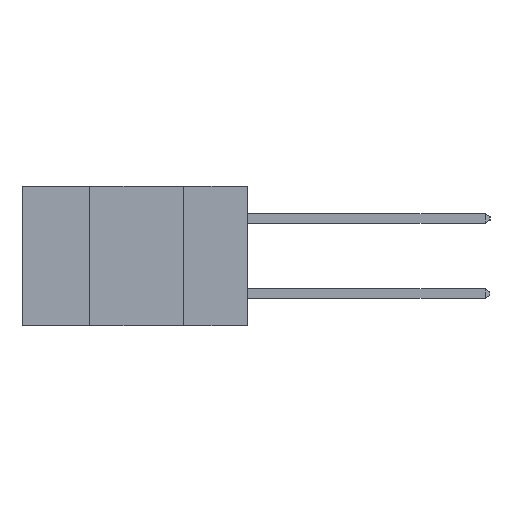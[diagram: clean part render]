
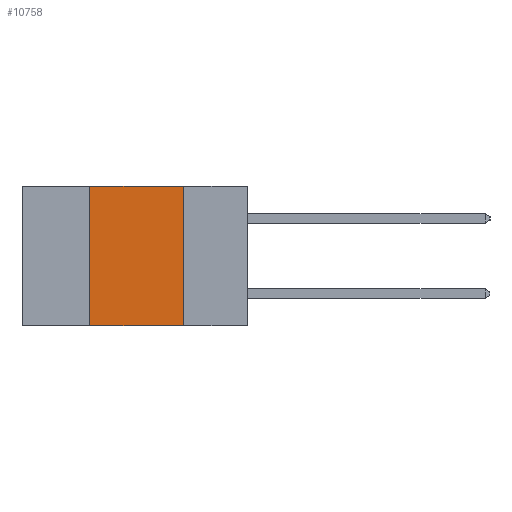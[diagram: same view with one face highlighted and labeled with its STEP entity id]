
A CAD part, left-side view. The second image highlights one B-rep face of the part: STEP entity #10758.
In plain terms, the highlighted planar face has unit normal (-1, 0, 0).
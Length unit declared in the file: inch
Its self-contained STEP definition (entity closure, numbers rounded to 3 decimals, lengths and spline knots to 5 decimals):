
#1154 = VERTEX_POINT ( 'NONE', #9420 ) ;
#1425 = CARTESIAN_POINT ( 'NONE',  ( 0., 0.17, 0. ) ) ;
#1762 = VERTEX_POINT ( 'NONE', #4291 ) ;
#2088 = CARTESIAN_POINT ( 'NONE',  ( 0., 0.42, 0. ) ) ;
#2187 = DIRECTION ( 'NONE',  ( 0., 0., 1. ) ) ;
#2316 = LINE ( 'NONE', #3023, #7748 ) ;
#2610 = LINE ( 'NONE', #6621, #13766 ) ;
#3023 = CARTESIAN_POINT ( 'NONE',  ( 0., 0.6, -0.37 ) ) ;
#3049 = ORIENTED_EDGE ( 'NONE', *, *, #9093, .F. ) ;
#3089 = VECTOR ( 'NONE', #7909, 39.37008 ) ;
#3754 = EDGE_LOOP ( 'NONE', ( #3049, #11776, #13810, #10653 ) ) ;
#3942 = LINE ( 'NONE', #8680, #7203 ) ;
#4291 = CARTESIAN_POINT ( 'NONE',  ( 0., 0.17, 0. ) ) ;
#4321 = DIRECTION ( 'NONE',  ( 0., 0., -1. ) ) ;
#4367 = VERTEX_POINT ( 'NONE', #2088 ) ;
#5024 = FACE_OUTER_BOUND ( 'NONE', #3754, .T. ) ;
#6621 = CARTESIAN_POINT ( 'NONE',  ( 0., 0.6, 0. ) ) ;
#6775 = CARTESIAN_POINT ( 'NONE',  ( 0., 0.6, 0. ) ) ;
#7203 = VECTOR ( 'NONE', #2187, 39.37008 ) ;
#7724 = DIRECTION ( 'NONE',  ( 0., -1., 0. ) ) ;
#7748 = VECTOR ( 'NONE', #11708, 39.37008 ) ;
#7909 = DIRECTION ( 'NONE',  ( 0., 0., -1. ) ) ;
#8337 = EDGE_CURVE ( 'NONE', #9006, #4367, #3942, .T. ) ;
#8441 = EDGE_CURVE ( 'NONE', #4367, #1762, #2610, .T. ) ;
#8680 = CARTESIAN_POINT ( 'NONE',  ( 0., 0.42, 0. ) ) ;
#8872 = CARTESIAN_POINT ( 'NONE',  ( 0., 0.42, -0.37 ) ) ;
#8896 = LINE ( 'NONE', #1425, #3089 ) ;
#9006 = VERTEX_POINT ( 'NONE', #8872 ) ;
#9093 = EDGE_CURVE ( 'NONE', #1762, #1154, #8896, .T. ) ;
#9420 = CARTESIAN_POINT ( 'NONE',  ( 0., 0.17, -0.37 ) ) ;
#9789 = PLANE ( 'NONE',  #12503 ) ;
#10653 = ORIENTED_EDGE ( 'NONE', *, *, #11854, .T. ) ;
#10758 = ADVANCED_FACE ( 'NONE', ( #5024 ), #9789, .F. ) ;
#10835 = DIRECTION ( 'NONE',  ( 1., 0., 0. ) ) ;
#11708 = DIRECTION ( 'NONE',  ( 0., -1., 0. ) ) ;
#11776 = ORIENTED_EDGE ( 'NONE', *, *, #8441, .F. ) ;
#11854 = EDGE_CURVE ( 'NONE', #9006, #1154, #2316, .T. ) ;
#12503 = AXIS2_PLACEMENT_3D ( 'NONE', #6775, #10835, #4321 ) ;
#13766 = VECTOR ( 'NONE', #7724, 39.37008 ) ;
#13810 = ORIENTED_EDGE ( 'NONE', *, *, #8337, .F. ) ;
